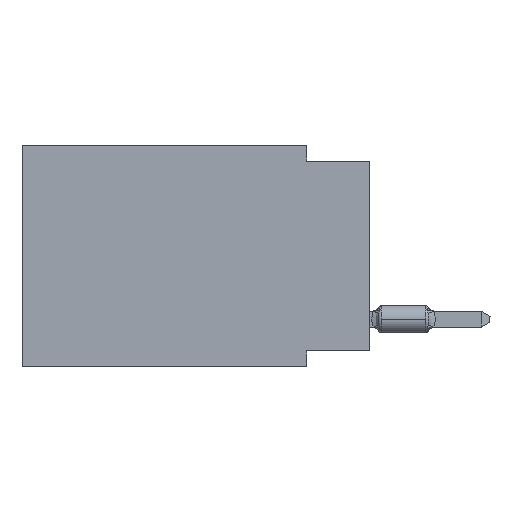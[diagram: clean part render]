
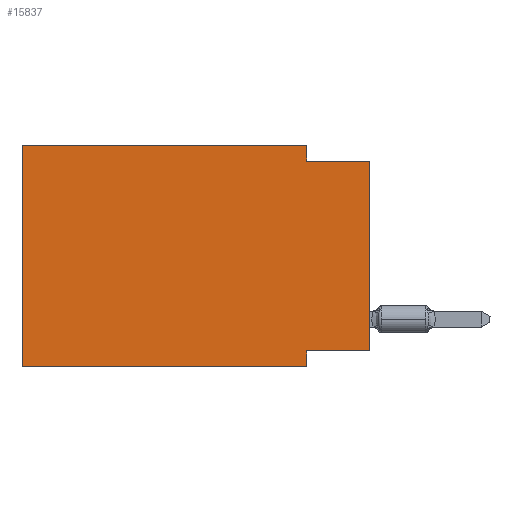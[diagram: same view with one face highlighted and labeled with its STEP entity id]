
A CAD part, left-side view. The second image highlights one B-rep face of the part: STEP entity #15837.
In plain terms, the highlighted planar face has unit normal (-1, 0, 0).
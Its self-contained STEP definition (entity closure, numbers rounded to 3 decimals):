
#273 = CARTESIAN_POINT ( 'NONE',  ( 0., 13.97, 0. ) ) ;
#1715 = CARTESIAN_POINT ( 'NONE',  ( 0., 13.97, 0. ) ) ;
#5382 = CARTESIAN_POINT ( 'NONE',  ( 0., 0., 0. ) ) ;
#5494 = CARTESIAN_POINT ( 'NONE',  ( 0., 13.97, 0. ) ) ;
#6184 = EDGE_CURVE ( 'NONE', #38894, #61211, #12818, .T. ) ;
#7109 = CARTESIAN_POINT ( 'NONE',  ( 0., 2.54, -8.255 ) ) ;
#11109 = VECTOR ( 'NONE', #80797, 1000. ) ;
#12765 = VERTEX_POINT ( 'NONE', #5494 ) ;
#12818 = LINE ( 'NONE', #53531, #83798 ) ;
#14037 = CARTESIAN_POINT ( 'NONE',  ( 0., 0., -8.255 ) ) ;
#14505 = VECTOR ( 'NONE', #75008, 1000. ) ;
#15594 = VERTEX_POINT ( 'NONE', #14037 ) ;
#15644 = CARTESIAN_POINT ( 'NONE',  ( 0., 2.54, -8.89 ) ) ;
#15837 = ADVANCED_FACE ( 'NONE', ( #35064 ), #62976, .F. ) ;
#18227 = LINE ( 'NONE', #5382, #33134 ) ;
#18561 = CARTESIAN_POINT ( 'NONE',  ( 0., 2.54, -8.89 ) ) ;
#18693 = CARTESIAN_POINT ( 'NONE',  ( 0., 0., -8.255 ) ) ;
#19265 = EDGE_CURVE ( 'NONE', #47851, #38894, #37786, .T. ) ;
#21189 = ORIENTED_EDGE ( 'NONE', *, *, #19265, .F. ) ;
#21427 = LINE ( 'NONE', #1715, #61406 ) ;
#22550 = AXIS2_PLACEMENT_3D ( 'NONE', #273, #28197, #56118 ) ;
#25720 = CARTESIAN_POINT ( 'NONE',  ( 0., 13.97, -8.89 ) ) ;
#26953 = EDGE_CURVE ( 'NONE', #81687, #77768, #88419, .T. ) ;
#28197 = DIRECTION ( 'NONE',  ( 1., 0., 0. ) ) ;
#29620 = DIRECTION ( 'NONE',  ( 0., 0., 1. ) ) ;
#29962 = ORIENTED_EDGE ( 'NONE', *, *, #26953, .T. ) ;
#30390 = EDGE_CURVE ( 'NONE', #12765, #47851, #90109, .T. ) ;
#33134 = VECTOR ( 'NONE', #46568, 1000. ) ;
#35064 = FACE_OUTER_BOUND ( 'NONE', #90321, .T. ) ;
#35594 = CARTESIAN_POINT ( 'NONE',  ( 0., 2.54, -0.635 ) ) ;
#37108 = LINE ( 'NONE', #15644, #71452 ) ;
#37786 = LINE ( 'NONE', #65245, #11109 ) ;
#38894 = VERTEX_POINT ( 'NONE', #35594 ) ;
#40637 = EDGE_CURVE ( 'NONE', #81687, #12765, #21427, .T. ) ;
#41274 = ORIENTED_EDGE ( 'NONE', *, *, #68378, .F. ) ;
#46568 = DIRECTION ( 'NONE',  ( 0., 0., 1. ) ) ;
#47851 = VERTEX_POINT ( 'NONE', #63236 ) ;
#48764 = VECTOR ( 'NONE', #82268, 1000. ) ;
#51675 = ORIENTED_EDGE ( 'NONE', *, *, #6184, .F. ) ;
#53531 = CARTESIAN_POINT ( 'NONE',  ( 0., 0., -0.635 ) ) ;
#53635 = DIRECTION ( 'NONE',  ( 0., -1., 0. ) ) ;
#54865 = CARTESIAN_POINT ( 'NONE',  ( 0., 13.97, 0. ) ) ;
#56118 = DIRECTION ( 'NONE',  ( 0., 0., -1. ) ) ;
#59305 = VERTEX_POINT ( 'NONE', #7109 ) ;
#60762 = LINE ( 'NONE', #18693, #48764 ) ;
#61211 = VERTEX_POINT ( 'NONE', #85132 ) ;
#61406 = VECTOR ( 'NONE', #29620, 1000. ) ;
#62825 = ORIENTED_EDGE ( 'NONE', *, *, #30390, .F. ) ;
#62976 = PLANE ( 'NONE',  #22550 ) ;
#63236 = CARTESIAN_POINT ( 'NONE',  ( 0., 2.54, 0. ) ) ;
#64832 = ORIENTED_EDGE ( 'NONE', *, *, #40637, .F. ) ;
#64956 = CARTESIAN_POINT ( 'NONE',  ( 0., 13.97, -8.89 ) ) ;
#65245 = CARTESIAN_POINT ( 'NONE',  ( 0., 2.54, 0. ) ) ;
#68378 = EDGE_CURVE ( 'NONE', #59305, #77768, #37108, .T. ) ;
#69412 = ORIENTED_EDGE ( 'NONE', *, *, #80147, .F. ) ;
#71452 = VECTOR ( 'NONE', #72343, 1000. ) ;
#72343 = DIRECTION ( 'NONE',  ( 0., 0., -1. ) ) ;
#75008 = DIRECTION ( 'NONE',  ( 0., -1., 0. ) ) ;
#77386 = EDGE_CURVE ( 'NONE', #15594, #61211, #18227, .T. ) ;
#77768 = VERTEX_POINT ( 'NONE', #18561 ) ;
#80147 = EDGE_CURVE ( 'NONE', #15594, #59305, #60762, .T. ) ;
#80580 = DIRECTION ( 'NONE',  ( 0., -1., 0. ) ) ;
#80797 = DIRECTION ( 'NONE',  ( 0., 0., -1. ) ) ;
#81267 = VECTOR ( 'NONE', #53635, 1000. ) ;
#81687 = VERTEX_POINT ( 'NONE', #64956 ) ;
#82268 = DIRECTION ( 'NONE',  ( 0., 1., 0. ) ) ;
#83798 = VECTOR ( 'NONE', #80580, 1000. ) ;
#85132 = CARTESIAN_POINT ( 'NONE',  ( 0., 0., -0.635 ) ) ;
#87715 = ORIENTED_EDGE ( 'NONE', *, *, #77386, .T. ) ;
#88419 = LINE ( 'NONE', #25720, #81267 ) ;
#90109 = LINE ( 'NONE', #54865, #14505 ) ;
#90321 = EDGE_LOOP ( 'NONE', ( #87715, #51675, #21189, #62825, #64832, #29962, #41274, #69412 ) ) ;
